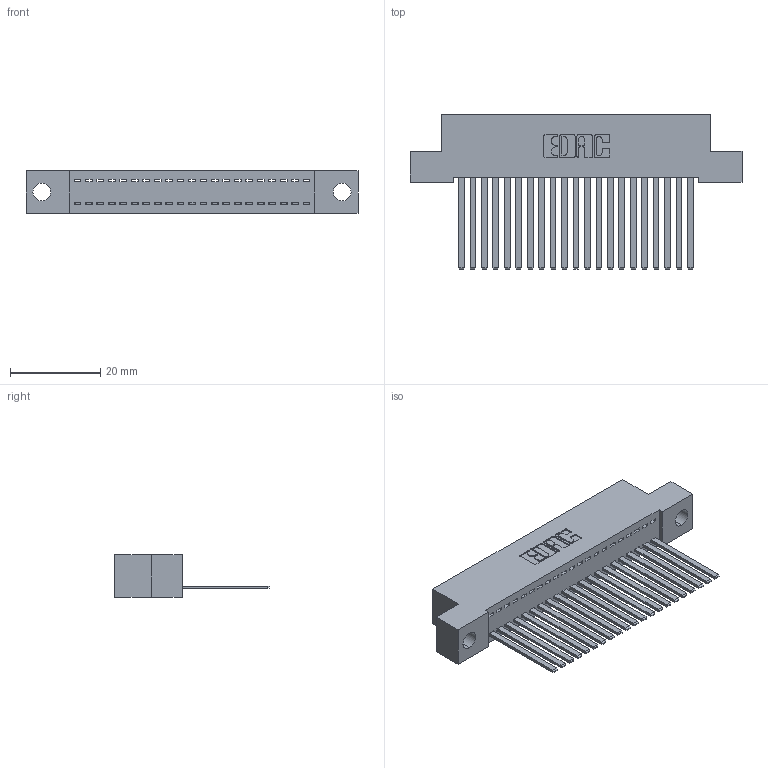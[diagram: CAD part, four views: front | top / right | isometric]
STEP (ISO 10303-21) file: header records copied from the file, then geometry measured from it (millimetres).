
FILE_DESCRIPTION (( 'STEP AP203' ), '1' );
FILE_NAME ('392-021-544-104.STEP', '2019-10-07T05:50:08', ( '' ), ( '' ), 'SwSTEP 2.0', 'SolidWorks 2016', '' );
FILE_SCHEMA (( 'CONFIG_CONTROL_DESIGN' ));
Length unit declared in the file: inch
Products named in the file (3): 342 Part_.156 TH; 345-292-001_345-293-144; 392-021-544-104
Assembly tree (22 placements, depth 2):
  392-021-544-104
    342 Part_.156 TH
    345-292-001_345-293-144  x21
Bounding box: 73.66 x 34.3 x 9.4 mm (x, y, z)
Volume: 6537.3 mm3; surface area: 9718.7 mm2
Topology: 22 solids, 22 shells, 1202 faces, 3617 edges, 2382 vertices
Faces by surface type: plane 864, cylinder 338
Entity records: 15241 total; most frequent: CARTESIAN_POINT 2637, ORIENTED_EDGE 2594, DIRECTION 2263, EDGE_CURVE 1297, LINE 1173, VECTOR 1173, VERTEX_POINT 862, AXIS2_PLACEMENT_3D 545
